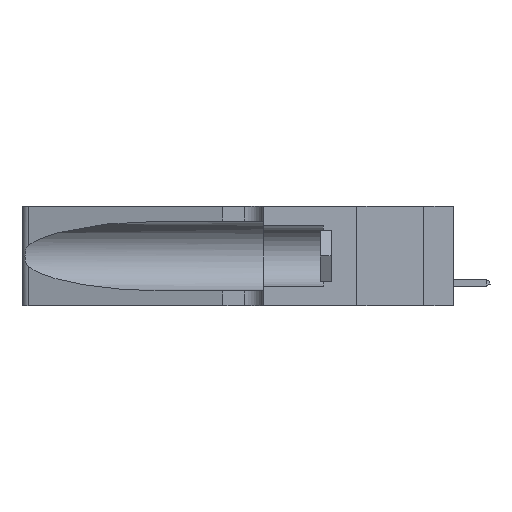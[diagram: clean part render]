
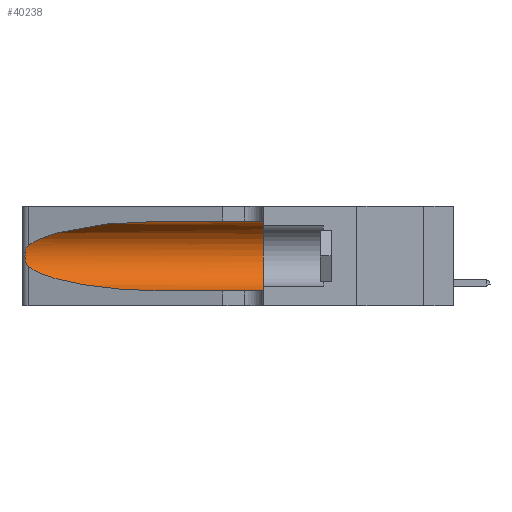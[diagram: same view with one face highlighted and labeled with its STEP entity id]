
A CAD part, left-side view. The second image highlights one B-rep face of the part: STEP entity #40238.
In plain terms, the highlighted cylindrical face has radius 3.308 mm (diameter 6.617 mm), a partial arc.
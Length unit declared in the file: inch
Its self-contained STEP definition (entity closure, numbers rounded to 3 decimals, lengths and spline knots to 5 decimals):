
#152 = CARTESIAN_POINT ( 'NONE',  ( 0.2373, 1.15595, 0.28018 ) ) ;
#905 = CARTESIAN_POINT ( 'NONE',  ( 0.26075, 1.23896, 0.178 ) ) ;
#1246 = CARTESIAN_POINT ( 'NONE',  ( 0.26075, 1.23896, 0.19203 ) ) ;
#2910 = EDGE_LOOP ( 'NONE', ( #34893, #25853, #42635, #14838, #5368, #32877 ) ) ;
#4379 = CARTESIAN_POINT ( 'NONE',  ( 0.26018, 1.23835, 0.19895 ) ) ;
#4842 = VERTEX_POINT ( 'NONE', #31676 ) ;
#4865 = CARTESIAN_POINT ( 'NONE',  ( 0.25555, 1.22993, 0.14849 ) ) ;
#5160 = DIRECTION ( 'NONE',  ( 0., 0., -1. ) ) ;
#5368 = ORIENTED_EDGE ( 'NONE', *, *, #24540, .F. ) ;
#5547 = DIRECTION ( 'NONE',  ( 0., 1., 0. ) ) ;
#5818 = EDGE_CURVE ( 'NONE', #18744, #40475, #5882, .T. ) ;
#5882 =( BOUNDED_CURVE ( )  B_SPLINE_CURVE ( 3, ( #18562, #29671, #29821, #15406 ),
 .UNSPECIFIED., .F., .F. ) 
 B_SPLINE_CURVE_WITH_KNOTS ( ( 4, 4 ),
 ( 3.44316, 4.71239 ),
 .UNSPECIFIED. ) 
 CURVE ( )  GEOMETRIC_REPRESENTATION_ITEM ( )  RATIONAL_B_SPLINE_CURVE ( ( 1., 0.87, 0.87, 1. ) ) 
 REPRESENTATION_ITEM ( '' )  );
#7526 = CARTESIAN_POINT ( 'NONE',  ( 0.18966, 0.96281, 0.31525 ) ) ;
#8161 = CARTESIAN_POINT ( 'NONE',  ( 0.25856, 1.23593, 0.16098 ) ) ;
#11890 = VERTEX_POINT ( 'NONE', #42792 ) ;
#12089 = VERTEX_POINT ( 'NONE', #21300 ) ;
#12139 = CARTESIAN_POINT ( 'NONE',  ( 0.1305, 0.35, 0.185 ) ) ;
#12432 = CIRCLE ( 'NONE', #35439, 0.13025 ) ;
#12942 = VECTOR ( 'NONE', #44393, 39.37008 ) ;
#13478 = VERTEX_POINT ( 'NONE', #28628 ) ;
#14232 = CARTESIAN_POINT ( 'NONE',  ( 0.25487, 1.22718, 0.22369 ) ) ;
#14383 = CARTESIAN_POINT ( 'NONE',  ( 0.1305, 0.72297, 0.31525 ) ) ;
#14838 = ORIENTED_EDGE ( 'NONE', *, *, #26669, .T. ) ;
#15261 = CARTESIAN_POINT ( 'NONE',  ( 0.25789, 1.23486, 0.15765 ) ) ;
#15406 = CARTESIAN_POINT ( 'NONE',  ( 0.1305, 0.72297, 0.05475 ) ) ;
#15771 = CARTESIAN_POINT ( 'NONE',  ( 0.25639, 1.23184, 0.21858 ) ) ;
#16291 = DIRECTION ( 'NONE',  ( 0., 0., 1. ) ) ;
#18017 = CARTESIAN_POINT ( 'NONE',  ( 0.25487, 1.22718, 0.22369 ) ) ;
#18562 = CARTESIAN_POINT ( 'NONE',  ( 0.25487, 1.22718, 0.14631 ) ) ;
#18744 = VERTEX_POINT ( 'NONE', #35920 ) ;
#19818 = EDGE_CURVE ( 'NONE', #4842, #11890, #28769, .T. ) ;
#21300 = CARTESIAN_POINT ( 'NONE',  ( 0.1305, 0.35, 0.05475 ) ) ;
#22237 = CARTESIAN_POINT ( 'NONE',  ( 0.25787, 1.23484, 0.2124 ) ) ;
#24540 = EDGE_CURVE ( 'NONE', #11890, #12089, #12432, .T. ) ;
#25141 = CARTESIAN_POINT ( 'NONE',  ( 0.25555, 1.22994, 0.2215 ) ) ;
#25294 = VECTOR ( 'NONE', #29304, 39.37008 ) ;
#25853 = ORIENTED_EDGE ( 'NONE', *, *, #30574, .T. ) ;
#26089 = B_SPLINE_CURVE_WITH_KNOTS ( 'NONE', 3,
 ( #18017, #25141, #15771, #22237, #40691, #4379, #1246, #905, #26506, #8161, #15261, #33669, #4865, #44297 ),
 .UNSPECIFIED., .F., .F.,
 ( 4, 2, 2, 2, 2, 2, 4 ),
 ( 0., 0.00027, 0.00053, 0.00107, 0.0016, 0.00187, 0.00214 ),
 .UNSPECIFIED. ) ;
#26506 = CARTESIAN_POINT ( 'NONE',  ( 0.26017, 1.23833, 0.17102 ) ) ;
#26669 = EDGE_CURVE ( 'NONE', #40475, #12089, #37261, .T. ) ;
#27523 = FACE_OUTER_BOUND ( 'NONE', #2910, .T. ) ;
#27913 = AXIS2_PLACEMENT_3D ( 'NONE', #40819, #40976, #5160 ) ;
#28628 = CARTESIAN_POINT ( 'NONE',  ( 0.25487, 1.22718, 0.22369 ) ) ;
#28769 = LINE ( 'NONE', #39996, #25294 ) ;
#29304 = DIRECTION ( 'NONE',  ( 0., -1., 0. ) ) ;
#29671 = CARTESIAN_POINT ( 'NONE',  ( 0.2373, 1.15595, 0.08982 ) ) ;
#29821 = CARTESIAN_POINT ( 'NONE',  ( 0.18966, 0.96281, 0.05475 ) ) ;
#30574 = EDGE_CURVE ( 'NONE', #13478, #18744, #26089, .T. ) ;
#31676 = CARTESIAN_POINT ( 'NONE',  ( 0.1305, 0.72297, 0.31525 ) ) ;
#32877 = ORIENTED_EDGE ( 'NONE', *, *, #19818, .F. ) ;
#33432 = CARTESIAN_POINT ( 'NONE',  ( 0.1305, 1.61858, 0.05475 ) ) ;
#33669 = CARTESIAN_POINT ( 'NONE',  ( 0.25639, 1.23186, 0.15144 ) ) ;
#34893 = ORIENTED_EDGE ( 'NONE', *, *, #42011, .T. ) ;
#35439 = AXIS2_PLACEMENT_3D ( 'NONE', #12139, #5547, #16291 ) ;
#35920 = CARTESIAN_POINT ( 'NONE',  ( 0.25487, 1.22718, 0.14631 ) ) ;
#36072 = CYLINDRICAL_SURFACE ( 'NONE', #27913, 0.13025 ) ;
#37261 = LINE ( 'NONE', #33432, #12942 ) ;
#39996 = CARTESIAN_POINT ( 'NONE',  ( 0.1305, 1.61858, 0.31525 ) ) ;
#40238 = ADVANCED_FACE ( 'NONE', ( #27523 ), #36072, .F. ) ;
#40475 = VERTEX_POINT ( 'NONE', #46226 ) ;
#40691 = CARTESIAN_POINT ( 'NONE',  ( 0.25854, 1.2359, 0.20912 ) ) ;
#40819 = CARTESIAN_POINT ( 'NONE',  ( 0.1305, 1.61858, 0.185 ) ) ;
#40976 = DIRECTION ( 'NONE',  ( 0., -1., 0. ) ) ;
#42011 = EDGE_CURVE ( 'NONE', #4842, #13478, #46572, .T. ) ;
#42635 = ORIENTED_EDGE ( 'NONE', *, *, #5818, .T. ) ;
#42792 = CARTESIAN_POINT ( 'NONE',  ( 0.1305, 0.35, 0.31525 ) ) ;
#44297 = CARTESIAN_POINT ( 'NONE',  ( 0.25487, 1.22718, 0.14631 ) ) ;
#44393 = DIRECTION ( 'NONE',  ( 0., -1., 0. ) ) ;
#46226 = CARTESIAN_POINT ( 'NONE',  ( 0.1305, 0.72297, 0.05475 ) ) ;
#46572 =( BOUNDED_CURVE ( )  B_SPLINE_CURVE ( 3, ( #14383, #7526, #152, #14232 ),
 .UNSPECIFIED., .F., .F. ) 
 B_SPLINE_CURVE_WITH_KNOTS ( ( 4, 4 ),
 ( 1.5708, 2.84003 ),
 .UNSPECIFIED. ) 
 CURVE ( )  GEOMETRIC_REPRESENTATION_ITEM ( )  RATIONAL_B_SPLINE_CURVE ( ( 1., 0.87, 0.87, 1. ) ) 
 REPRESENTATION_ITEM ( '' )  );
